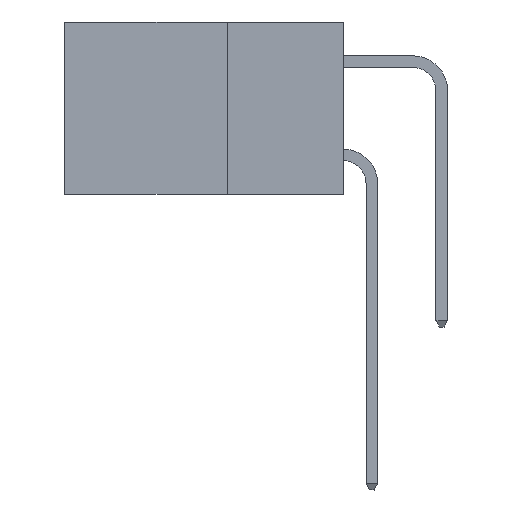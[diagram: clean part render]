
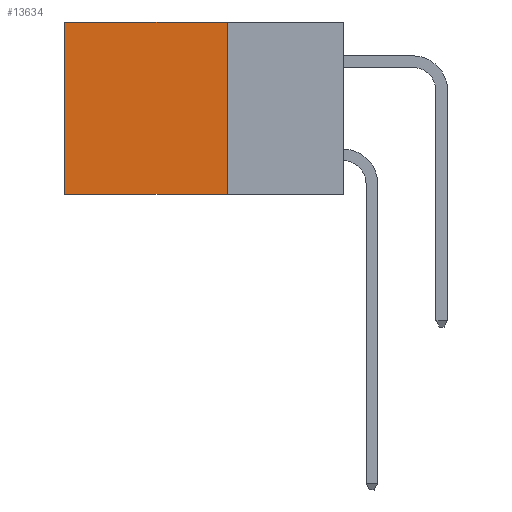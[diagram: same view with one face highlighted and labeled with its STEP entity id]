
A CAD part, left-side view. The second image highlights one B-rep face of the part: STEP entity #13634.
In plain terms, the highlighted planar face has unit normal (-1, 0, 0).
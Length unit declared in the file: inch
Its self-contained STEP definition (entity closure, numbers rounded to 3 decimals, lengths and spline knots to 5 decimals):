
#586 = CARTESIAN_POINT ( 'NONE',  ( 0.298, 0.6, 0. ) ) ;
#1052 = DIRECTION ( 'NONE',  ( 1., 0., 0. ) ) ;
#1871 = DIRECTION ( 'NONE',  ( 0., 0., -1. ) ) ;
#2413 = VERTEX_POINT ( 'NONE', #14830 ) ;
#2799 = DIRECTION ( 'NONE',  ( 0., 1., 0. ) ) ;
#3357 = LINE ( 'NONE', #10962, #9891 ) ;
#4306 = ORIENTED_EDGE ( 'NONE', *, *, #13724, .T. ) ;
#5177 = DIRECTION ( 'NONE',  ( 0., 1., 0. ) ) ;
#5382 = ORIENTED_EDGE ( 'NONE', *, *, #7032, .T. ) ;
#6452 = LINE ( 'NONE', #11085, #17144 ) ;
#7032 = EDGE_CURVE ( 'NONE', #14395, #8796, #10735, .T. ) ;
#8763 = VECTOR ( 'NONE', #13632, 39.37008 ) ;
#8796 = VERTEX_POINT ( 'NONE', #15434 ) ;
#9263 = VECTOR ( 'NONE', #1871, 39.37008 ) ;
#9338 = DIRECTION ( 'NONE',  ( 0., 0., -1. ) ) ;
#9891 = VECTOR ( 'NONE', #5177, 39.37008 ) ;
#10174 = CARTESIAN_POINT ( 'NONE',  ( 0.298, 0.25, 0. ) ) ;
#10735 = LINE ( 'NONE', #17725, #8763 ) ;
#10895 = VERTEX_POINT ( 'NONE', #10174 ) ;
#10962 = CARTESIAN_POINT ( 'NONE',  ( 0.298, 0.25, -0.37 ) ) ;
#11085 = CARTESIAN_POINT ( 'NONE',  ( 0.298, 0.25, 0. ) ) ;
#12284 = ORIENTED_EDGE ( 'NONE', *, *, #13331, .F. ) ;
#12842 = ORIENTED_EDGE ( 'NONE', *, *, #14679, .F. ) ;
#12999 = FACE_OUTER_BOUND ( 'NONE', #15503, .T. ) ;
#13331 = EDGE_CURVE ( 'NONE', #10895, #2413, #17801, .T. ) ;
#13632 = DIRECTION ( 'NONE',  ( 0., 0., -1. ) ) ;
#13634 = ADVANCED_FACE ( 'NONE', ( #12999 ), #17731, .F. ) ;
#13724 = EDGE_CURVE ( 'NONE', #10895, #14395, #6452, .T. ) ;
#14395 = VERTEX_POINT ( 'NONE', #586 ) ;
#14512 = AXIS2_PLACEMENT_3D ( 'NONE', #14805, #1052, #9338 ) ;
#14679 = EDGE_CURVE ( 'NONE', #2413, #8796, #3357, .T. ) ;
#14805 = CARTESIAN_POINT ( 'NONE',  ( 0.298, 0.25, 0. ) ) ;
#14830 = CARTESIAN_POINT ( 'NONE',  ( 0.298, 0.25, -0.37 ) ) ;
#15434 = CARTESIAN_POINT ( 'NONE',  ( 0.298, 0.6, -0.37 ) ) ;
#15503 = EDGE_LOOP ( 'NONE', ( #5382, #12842, #12284, #4306 ) ) ;
#17076 = CARTESIAN_POINT ( 'NONE',  ( 0.298, 0.25, 0. ) ) ;
#17144 = VECTOR ( 'NONE', #2799, 39.37008 ) ;
#17725 = CARTESIAN_POINT ( 'NONE',  ( 0.298, 0.6, 0. ) ) ;
#17731 = PLANE ( 'NONE',  #14512 ) ;
#17801 = LINE ( 'NONE', #17076, #9263 ) ;
